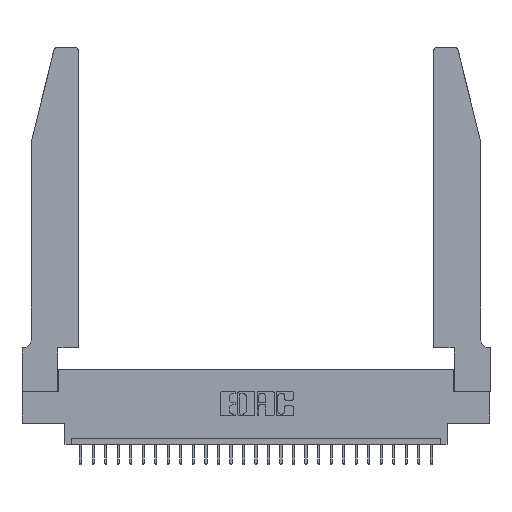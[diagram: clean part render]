
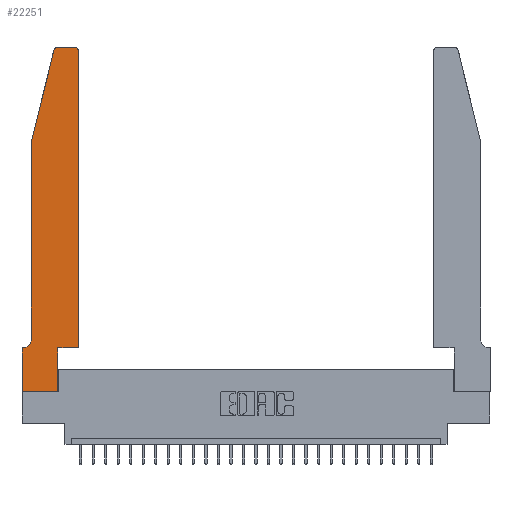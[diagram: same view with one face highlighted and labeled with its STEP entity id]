
A CAD part, top view. The second image highlights one B-rep face of the part: STEP entity #22251.
In plain terms, the highlighted planar face has unit normal (0, 0, 1).
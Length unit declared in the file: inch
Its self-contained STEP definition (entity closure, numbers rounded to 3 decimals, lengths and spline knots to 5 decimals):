
#72 = CARTESIAN_POINT ( 'NONE',  ( 0., 0.35, 0.37 ) ) ;
#75 = ORIENTED_EDGE ( 'NONE', *, *, #3583, .T. ) ;
#381 = LINE ( 'NONE', #15208, #26941 ) ;
#1292 = CARTESIAN_POINT ( 'NONE',  ( 0.0755, 0.35, 0.37 ) ) ;
#1671 = EDGE_CURVE ( 'NONE', #17079, #27843, #15350, .T. ) ;
#1792 = CIRCLE ( 'NONE', #10347, 0.03 ) ;
#1879 = DIRECTION ( 'NONE',  ( 1., 0., 0. ) ) ;
#2052 = CARTESIAN_POINT ( 'NONE',  ( 0.2865, 0., 0.37 ) ) ;
#2497 = CARTESIAN_POINT ( 'NONE',  ( 0., 0., 0.37 ) ) ;
#3129 = FACE_OUTER_BOUND ( 'NONE', #4778, .T. ) ;
#3305 = DIRECTION ( 'NONE',  ( 0., -1., 0. ) ) ;
#3390 = LINE ( 'NONE', #7978, #19644 ) ;
#3489 = EDGE_CURVE ( 'NONE', #27843, #10938, #25990, .T. ) ;
#3573 = AXIS2_PLACEMENT_3D ( 'NONE', #72, #11094, #13303 ) ;
#3583 = EDGE_CURVE ( 'NONE', #10938, #26292, #25285, .T. ) ;
#3771 = DIRECTION ( 'NONE',  ( 0., 0., 1. ) ) ;
#4080 = EDGE_CURVE ( 'NONE', #22602, #20160, #381, .T. ) ;
#4224 = DIRECTION ( 'NONE',  ( -1., 0., 0. ) ) ;
#4481 = DIRECTION ( 'NONE',  ( -0.239, -0.971, 0. ) ) ;
#4778 = EDGE_LOOP ( 'NONE', ( #14831, #26517, #75, #6755, #28247, #15690, #17811, #11674, #15407, #17342, #25912, #9936 ) ) ;
#5237 = EDGE_CURVE ( 'NONE', #23481, #6717, #25450, .T. ) ;
#5503 = VERTEX_POINT ( 'NONE', #12966 ) ;
#5563 = CARTESIAN_POINT ( 'NONE',  ( 0.2605, 2.75, 0.37 ) ) ;
#6717 = VERTEX_POINT ( 'NONE', #2497 ) ;
#6755 = ORIENTED_EDGE ( 'NONE', *, *, #15514, .T. ) ;
#7325 = CARTESIAN_POINT ( 'NONE',  ( 0.4205, 2.75, 0.37 ) ) ;
#7640 = VERTEX_POINT ( 'NONE', #12379 ) ;
#7854 = VECTOR ( 'NONE', #12138, 39.37008 ) ;
#7978 = CARTESIAN_POINT ( 'NONE',  ( 0., 0., 0.37 ) ) ;
#7995 = CARTESIAN_POINT ( 'NONE',  ( 0.4505, 0.35, 0.37 ) ) ;
#8738 = DIRECTION ( 'NONE',  ( 0., 1., 0. ) ) ;
#9072 = DIRECTION ( 'NONE',  ( 1., 0., 0. ) ) ;
#9156 = DIRECTION ( 'NONE',  ( 0., 0., -1. ) ) ;
#9465 = CARTESIAN_POINT ( 'NONE',  ( 0.0755, 0.42, 0.37 ) ) ;
#9893 = EDGE_CURVE ( 'NONE', #5503, #17079, #1792, .T. ) ;
#9936 = ORIENTED_EDGE ( 'NONE', *, *, #9893, .T. ) ;
#10347 = AXIS2_PLACEMENT_3D ( 'NONE', #12840, #3771, #1879 ) ;
#10938 = VERTEX_POINT ( 'NONE', #19018 ) ;
#11017 = VERTEX_POINT ( 'NONE', #14909 ) ;
#11094 = DIRECTION ( 'NONE',  ( 0., 0., 1. ) ) ;
#11168 = EDGE_CURVE ( 'NONE', #11017, #23481, #19063, .T. ) ;
#11674 = ORIENTED_EDGE ( 'NONE', *, *, #13085, .T. ) ;
#11951 = DIRECTION ( 'NONE',  ( 0., -1., 0. ) ) ;
#11982 = CIRCLE ( 'NONE', #15641, 0.07 ) ;
#12138 = DIRECTION ( 'NONE',  ( 0., 1., 0. ) ) ;
#12379 = CARTESIAN_POINT ( 'NONE',  ( 0.4505, 0.35, 0.37 ) ) ;
#12840 = CARTESIAN_POINT ( 'NONE',  ( 0.4205, 2.72, 0.37 ) ) ;
#12966 = CARTESIAN_POINT ( 'NONE',  ( 0.4505, 2.72, 0.37 ) ) ;
#13046 = LINE ( 'NONE', #7995, #25838 ) ;
#13085 = EDGE_CURVE ( 'NONE', #6717, #22602, #3390, .T. ) ;
#13287 = LINE ( 'NONE', #22986, #25058 ) ;
#13303 = DIRECTION ( 'NONE',  ( 1., 0., 0. ) ) ;
#13617 = CARTESIAN_POINT ( 'NONE',  ( 0.0055, 0.42, 0.37 ) ) ;
#14078 = CARTESIAN_POINT ( 'NONE',  ( 0.284, 2.75, 0.37 ) ) ;
#14093 = EDGE_CURVE ( 'NONE', #27925, #11017, #11982, .T. ) ;
#14825 = DIRECTION ( 'NONE',  ( 1., 0., 0. ) ) ;
#14831 = ORIENTED_EDGE ( 'NONE', *, *, #1671, .T. ) ;
#14909 = CARTESIAN_POINT ( 'NONE',  ( 0.0055, 0.35, 0.37 ) ) ;
#15179 = DIRECTION ( 'NONE',  ( 0., 0., 1. ) ) ;
#15208 = CARTESIAN_POINT ( 'NONE',  ( 0.2865, 0.35, 0.37 ) ) ;
#15350 = LINE ( 'NONE', #5563, #20583 ) ;
#15407 = ORIENTED_EDGE ( 'NONE', *, *, #4080, .T. ) ;
#15514 = EDGE_CURVE ( 'NONE', #26292, #27925, #13287, .T. ) ;
#15641 = AXIS2_PLACEMENT_3D ( 'NONE', #13617, #9156, #18386 ) ;
#15690 = ORIENTED_EDGE ( 'NONE', *, *, #11168, .T. ) ;
#16514 = CARTESIAN_POINT ( 'NONE',  ( 0., 0., 0.37 ) ) ;
#17079 = VERTEX_POINT ( 'NONE', #7325 ) ;
#17342 = ORIENTED_EDGE ( 'NONE', *, *, #26333, .T. ) ;
#17811 = ORIENTED_EDGE ( 'NONE', *, *, #5237, .T. ) ;
#17977 = AXIS2_PLACEMENT_3D ( 'NONE', #21814, #15179, #9072 ) ;
#18386 = DIRECTION ( 'NONE',  ( -1., 0., 0. ) ) ;
#19018 = CARTESIAN_POINT ( 'NONE',  ( 0.25487, 2.72718, 0.37 ) ) ;
#19063 = LINE ( 'NONE', #1292, #20795 ) ;
#19644 = VECTOR ( 'NONE', #14825, 39.37008 ) ;
#20057 = CARTESIAN_POINT ( 'NONE',  ( 0.0755, 2., 0.37 ) ) ;
#20160 = VERTEX_POINT ( 'NONE', #26135 ) ;
#20583 = VECTOR ( 'NONE', #27694, 39.37008 ) ;
#20795 = VECTOR ( 'NONE', #4224, 39.37008 ) ;
#21070 = CARTESIAN_POINT ( 'NONE',  ( 0.0755, 2., 0.37 ) ) ;
#21168 = CARTESIAN_POINT ( 'NONE',  ( 0., 0.35, 0.37 ) ) ;
#21814 = CARTESIAN_POINT ( 'NONE',  ( 0.284, 2.72, 0.37 ) ) ;
#22251 = ADVANCED_FACE ( 'NONE', ( #3129 ), #24281, .T. ) ;
#22602 = VERTEX_POINT ( 'NONE', #2052 ) ;
#22878 = VECTOR ( 'NONE', #4481, 39.37008 ) ;
#22986 = CARTESIAN_POINT ( 'NONE',  ( 0.0755, 2., 0.37 ) ) ;
#23481 = VERTEX_POINT ( 'NONE', #21168 ) ;
#24281 = PLANE ( 'NONE',  #3573 ) ;
#25058 = VECTOR ( 'NONE', #11951, 39.37008 ) ;
#25285 = LINE ( 'NONE', #20057, #22878 ) ;
#25450 = LINE ( 'NONE', #16514, #26169 ) ;
#25678 = EDGE_CURVE ( 'NONE', #7640, #5503, #26244, .T. ) ;
#25838 = VECTOR ( 'NONE', #27815, 39.37008 ) ;
#25912 = ORIENTED_EDGE ( 'NONE', *, *, #25678, .T. ) ;
#25990 = CIRCLE ( 'NONE', #17977, 0.03 ) ;
#26135 = CARTESIAN_POINT ( 'NONE',  ( 0.2865, 0.35, 0.37 ) ) ;
#26169 = VECTOR ( 'NONE', #3305, 39.37008 ) ;
#26244 = LINE ( 'NONE', #27514, #7854 ) ;
#26292 = VERTEX_POINT ( 'NONE', #21070 ) ;
#26333 = EDGE_CURVE ( 'NONE', #20160, #7640, #13046, .T. ) ;
#26517 = ORIENTED_EDGE ( 'NONE', *, *, #3489, .T. ) ;
#26941 = VECTOR ( 'NONE', #8738, 39.37008 ) ;
#27514 = CARTESIAN_POINT ( 'NONE',  ( 0.4505, 0.35, 0.37 ) ) ;
#27694 = DIRECTION ( 'NONE',  ( -1., 0., 0. ) ) ;
#27815 = DIRECTION ( 'NONE',  ( 1., 0., 0. ) ) ;
#27843 = VERTEX_POINT ( 'NONE', #14078 ) ;
#27925 = VERTEX_POINT ( 'NONE', #9465 ) ;
#28247 = ORIENTED_EDGE ( 'NONE', *, *, #14093, .T. ) ;
